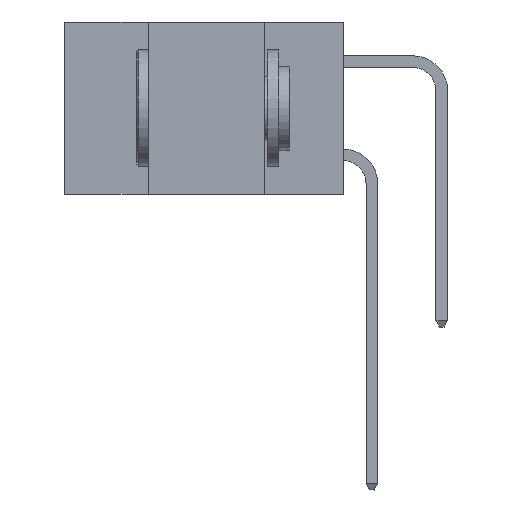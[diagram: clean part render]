
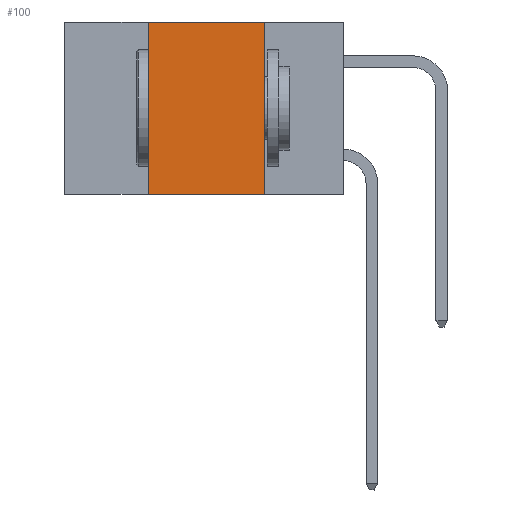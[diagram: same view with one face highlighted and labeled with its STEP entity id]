
A CAD part, left-side view. The second image highlights one B-rep face of the part: STEP entity #100.
In plain terms, the highlighted planar face has unit normal (-1, 0, 0).
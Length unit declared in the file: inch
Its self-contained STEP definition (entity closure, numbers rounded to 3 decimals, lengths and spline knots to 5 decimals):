
#33 = PLANE ( 'NONE',  #10669 ) ;
#100 = ADVANCED_FACE ( 'NONE', ( #14650 ), #33, .F. ) ;
#267 = CARTESIAN_POINT ( 'NONE',  ( 0., 0.17, 0. ) ) ;
#1509 = VECTOR ( 'NONE', #9762, 39.37008 ) ;
#1857 = EDGE_CURVE ( 'NONE', #7301, #8959, #2726, .T. ) ;
#2298 = VERTEX_POINT ( 'NONE', #13812 ) ;
#2726 = LINE ( 'NONE', #10911, #5738 ) ;
#2968 = LINE ( 'NONE', #8622, #12032 ) ;
#4914 = LINE ( 'NONE', #7295, #1509 ) ;
#5167 = EDGE_LOOP ( 'NONE', ( #14036, #12006, #12389, #6737 ) ) ;
#5354 = CARTESIAN_POINT ( 'NONE',  ( 0., 0.17, -0.37 ) ) ;
#5738 = VECTOR ( 'NONE', #7432, 39.37008 ) ;
#6481 = DIRECTION ( 'NONE',  ( 0., 0., -1. ) ) ;
#6559 = CARTESIAN_POINT ( 'NONE',  ( 0., 0.42, -0.37 ) ) ;
#6737 = ORIENTED_EDGE ( 'NONE', *, *, #1857, .T. ) ;
#6741 = DIRECTION ( 'NONE',  ( 0., 0., 1. ) ) ;
#7295 = CARTESIAN_POINT ( 'NONE',  ( 0., 0.6, 0. ) ) ;
#7301 = VERTEX_POINT ( 'NONE', #6559 ) ;
#7335 = VERTEX_POINT ( 'NONE', #267 ) ;
#7432 = DIRECTION ( 'NONE',  ( 0., -1., 0. ) ) ;
#8237 = LINE ( 'NONE', #13923, #14597 ) ;
#8622 = CARTESIAN_POINT ( 'NONE',  ( 0., 0.17, 0. ) ) ;
#8959 = VERTEX_POINT ( 'NONE', #5354 ) ;
#9725 = EDGE_CURVE ( 'NONE', #7301, #2298, #8237, .T. ) ;
#9762 = DIRECTION ( 'NONE',  ( 0., -1., 0. ) ) ;
#10304 = DIRECTION ( 'NONE',  ( 1., 0., 0. ) ) ;
#10598 = EDGE_CURVE ( 'NONE', #2298, #7335, #4914, .T. ) ;
#10669 = AXIS2_PLACEMENT_3D ( 'NONE', #15182, #10304, #6481 ) ;
#10911 = CARTESIAN_POINT ( 'NONE',  ( 0., 0.6, -0.37 ) ) ;
#12006 = ORIENTED_EDGE ( 'NONE', *, *, #10598, .F. ) ;
#12032 = VECTOR ( 'NONE', #14612, 39.37008 ) ;
#12389 = ORIENTED_EDGE ( 'NONE', *, *, #9725, .F. ) ;
#13812 = CARTESIAN_POINT ( 'NONE',  ( 0., 0.42, 0. ) ) ;
#13923 = CARTESIAN_POINT ( 'NONE',  ( 0., 0.42, 0. ) ) ;
#13978 = EDGE_CURVE ( 'NONE', #7335, #8959, #2968, .T. ) ;
#14036 = ORIENTED_EDGE ( 'NONE', *, *, #13978, .F. ) ;
#14597 = VECTOR ( 'NONE', #6741, 39.37008 ) ;
#14612 = DIRECTION ( 'NONE',  ( 0., 0., -1. ) ) ;
#14650 = FACE_OUTER_BOUND ( 'NONE', #5167, .T. ) ;
#15182 = CARTESIAN_POINT ( 'NONE',  ( 0., 0.6, 0. ) ) ;
